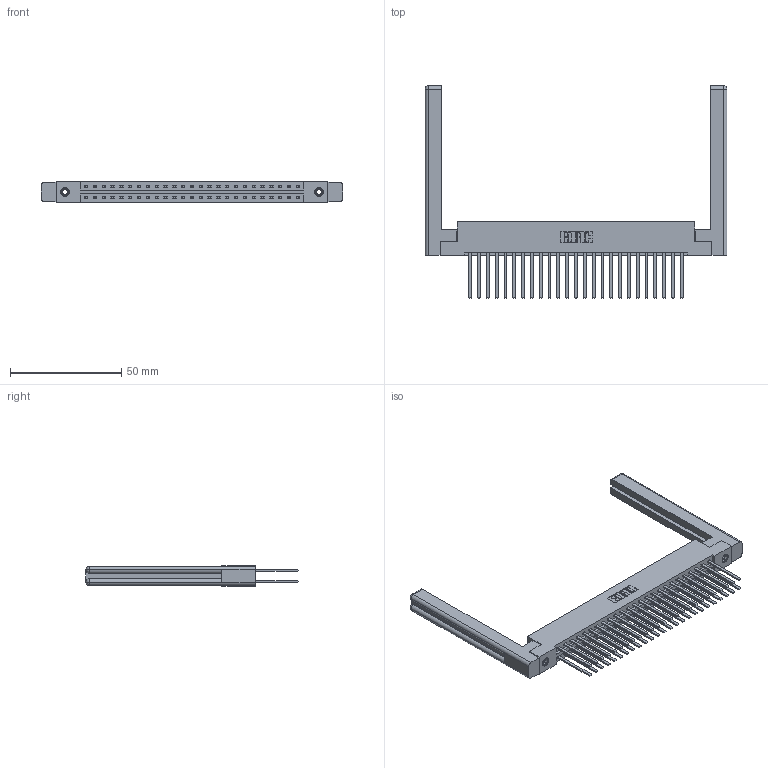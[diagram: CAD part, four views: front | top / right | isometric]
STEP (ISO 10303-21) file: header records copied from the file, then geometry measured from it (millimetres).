
FILE_DESCRIPTION (( 'STEP AP203' ), '1' );
FILE_NAME ('387-050-544-258.STEP', '2019-10-19T02:06:34', ( '' ), ( '' ), 'SwSTEP 2.0', 'SolidWorks 2016', '' );
FILE_SCHEMA (( 'CONFIG_CONTROL_DESIGN' ));
Length unit declared in the file: inch
Products named in the file (5): 345-250-001_345-250-001-102; 307-220-058; 387-050-544-258; 345-292-001_345-293-144; 337 Part_Flush Mounting Lugs - 0.156 Dia-TI
Assembly tree (55 placements, depth 2):
  387-050-544-258
    337 Part_Flush Mounting Lugs - 0.156 Dia-TI
    345-292-001_345-293-144  x50
    345-250-001_345-250-001-102  x2
    307-220-058  x2
Bounding box: 135.69 x 95.38 x 9.4 mm (x, y, z)
Volume: 21916.7 mm3; surface area: 23873.8 mm2
Topology: 55 solids, 55 shells, 2656 faces, 7815 edges, 5130 vertices
Faces by surface type: plane 1854, cylinder 778, cone 12, torus 12
Entity records: 24032 total; most frequent: CARTESIAN_POINT 4069, ORIENTED_EDGE 3944, DIRECTION 3504, EDGE_CURVE 1972, VECTOR 1800, LINE 1800, VERTEX_POINT 1306, AXIS2_PLACEMENT_3D 852
